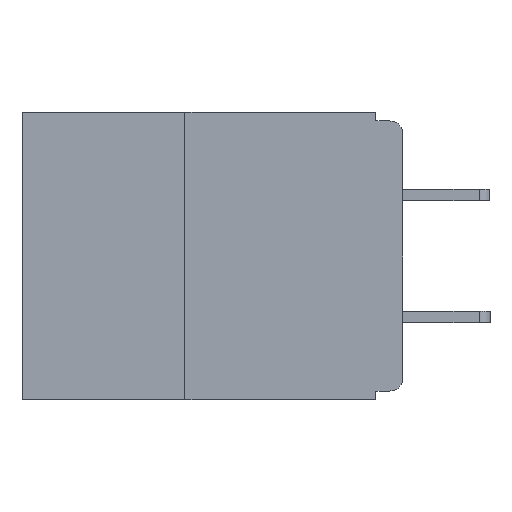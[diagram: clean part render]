
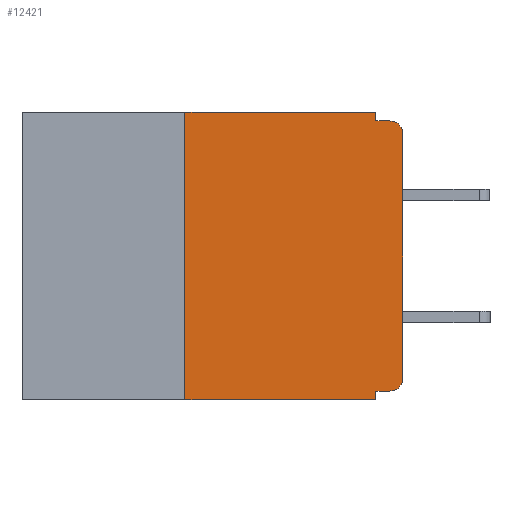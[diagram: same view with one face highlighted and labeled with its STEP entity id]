
A CAD part, left-side view. The second image highlights one B-rep face of the part: STEP entity #12421.
In plain terms, the highlighted planar face has unit normal (-1, 0, 0).
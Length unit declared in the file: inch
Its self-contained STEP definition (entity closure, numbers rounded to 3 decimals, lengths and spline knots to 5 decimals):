
#20 = ORIENTED_EDGE ( 'NONE', *, *, #16662, .T. ) ;
#504 = CARTESIAN_POINT ( 'NONE',  ( 0., 0., 0. ) ) ;
#861 = CARTESIAN_POINT ( 'NONE',  ( 0., 0., -0.025 ) ) ;
#1582 = ORIENTED_EDGE ( 'NONE', *, *, #31249, .T. ) ;
#1632 = VERTEX_POINT ( 'NONE', #21665 ) ;
#2095 = LINE ( 'NONE', #20295, #14384 ) ;
#2736 = AXIS2_PLACEMENT_3D ( 'NONE', #5740, #22915, #8243 ) ;
#3205 = CARTESIAN_POINT ( 'NONE',  ( 0., 0.031, -0.33 ) ) ;
#3583 = CARTESIAN_POINT ( 'NONE',  ( 0., 0.031, 0. ) ) ;
#3768 = VERTEX_POINT ( 'NONE', #4635 ) ;
#4081 = VECTOR ( 'NONE', #13681, 39.37008 ) ;
#4127 = DIRECTION ( 'NONE',  ( 0., 0., -1. ) ) ;
#4635 = CARTESIAN_POINT ( 'NONE',  ( 0., 0.015, -0.32 ) ) ;
#4846 = LINE ( 'NONE', #29127, #23642 ) ;
#5740 = CARTESIAN_POINT ( 'NONE',  ( 0., 0.015, -0.305 ) ) ;
#5940 = DIRECTION ( 'NONE',  ( 1., 0., 0. ) ) ;
#6138 = VERTEX_POINT ( 'NONE', #16312 ) ;
#6229 = CARTESIAN_POINT ( 'NONE',  ( 0., 0.015, -0.025 ) ) ;
#6965 = ORIENTED_EDGE ( 'NONE', *, *, #12370, .T. ) ;
#7021 = VERTEX_POINT ( 'NONE', #3205 ) ;
#7223 = FACE_OUTER_BOUND ( 'NONE', #7234, .T. ) ;
#7234 = EDGE_LOOP ( 'NONE', ( #1582, #16169, #7750, #20772, #28687, #18882, #20, #30564, #12710, #6965 ) ) ;
#7750 = ORIENTED_EDGE ( 'NONE', *, *, #13409, .F. ) ;
#8199 = EDGE_CURVE ( 'NONE', #6138, #17475, #31537, .T. ) ;
#8243 = DIRECTION ( 'NONE',  ( 0., 0., -1. ) ) ;
#8496 = LINE ( 'NONE', #3583, #25672 ) ;
#8737 = DIRECTION ( 'NONE',  ( 0., 0., -1. ) ) ;
#9565 = CIRCLE ( 'NONE', #2736, 0.015 ) ;
#9717 = VECTOR ( 'NONE', #4127, 39.37008 ) ;
#10098 = EDGE_CURVE ( 'NONE', #19013, #7021, #17009, .T. ) ;
#11985 = LINE ( 'NONE', #24478, #24993 ) ;
#12370 = EDGE_CURVE ( 'NONE', #3768, #24733, #9565, .T. ) ;
#12421 = ADVANCED_FACE ( 'NONE', ( #7223 ), #18208, .F. ) ;
#12710 = ORIENTED_EDGE ( 'NONE', *, *, #27077, .F. ) ;
#13221 = CARTESIAN_POINT ( 'NONE',  ( 0., 0.015, -0.01 ) ) ;
#13409 = EDGE_CURVE ( 'NONE', #1632, #30716, #4846, .T. ) ;
#13681 = DIRECTION ( 'NONE',  ( 0., -1., 0. ) ) ;
#14384 = VECTOR ( 'NONE', #22774, 39.37008 ) ;
#14956 = DIRECTION ( 'NONE',  ( 0., -1., 0. ) ) ;
#16169 = ORIENTED_EDGE ( 'NONE', *, *, #18958, .T. ) ;
#16205 = CARTESIAN_POINT ( 'NONE',  ( 0., 0.031, -0.32 ) ) ;
#16312 = CARTESIAN_POINT ( 'NONE',  ( 0., 0.25, 0. ) ) ;
#16662 = EDGE_CURVE ( 'NONE', #31439, #7021, #23657, .T. ) ;
#17009 = LINE ( 'NONE', #28443, #9717 ) ;
#17128 = DIRECTION ( 'NONE',  ( 0., 0., 1. ) ) ;
#17278 = VECTOR ( 'NONE', #17742, 39.37008 ) ;
#17475 = VERTEX_POINT ( 'NONE', #24228 ) ;
#17592 = AXIS2_PLACEMENT_3D ( 'NONE', #20644, #5940, #23116 ) ;
#17742 = DIRECTION ( 'NONE',  ( 0., 0., 1. ) ) ;
#18208 = PLANE ( 'NONE',  #17592 ) ;
#18221 = CARTESIAN_POINT ( 'NONE',  ( 0., 0., -0.305 ) ) ;
#18774 = VECTOR ( 'NONE', #14956, 39.37008 ) ;
#18882 = ORIENTED_EDGE ( 'NONE', *, *, #19933, .F. ) ;
#18958 = EDGE_CURVE ( 'NONE', #27129, #30716, #28365, .T. ) ;
#19013 = VERTEX_POINT ( 'NONE', #16205 ) ;
#19773 = CARTESIAN_POINT ( 'NONE',  ( 0., 0.437, 0. ) ) ;
#19933 = EDGE_CURVE ( 'NONE', #31439, #6138, #11985, .T. ) ;
#20295 = CARTESIAN_POINT ( 'NONE',  ( 0., 0., -0.32 ) ) ;
#20644 = CARTESIAN_POINT ( 'NONE',  ( 0., 0.437, 0. ) ) ;
#20747 = DIRECTION ( 'NONE',  ( 0., 0., -1. ) ) ;
#20772 = ORIENTED_EDGE ( 'NONE', *, *, #23218, .F. ) ;
#21665 = CARTESIAN_POINT ( 'NONE',  ( 0., 0.031, -0.01 ) ) ;
#22774 = DIRECTION ( 'NONE',  ( 0., 1., 0. ) ) ;
#22915 = DIRECTION ( 'NONE',  ( -1., 0., 0. ) ) ;
#23116 = DIRECTION ( 'NONE',  ( 0., 0., -1. ) ) ;
#23218 = EDGE_CURVE ( 'NONE', #17475, #1632, #8496, .T. ) ;
#23260 = CARTESIAN_POINT ( 'NONE',  ( 0., 0.25, -0.33 ) ) ;
#23377 = DIRECTION ( 'NONE',  ( -1., 0., 0. ) ) ;
#23642 = VECTOR ( 'NONE', #26746, 39.37008 ) ;
#23657 = LINE ( 'NONE', #25843, #4081 ) ;
#24228 = CARTESIAN_POINT ( 'NONE',  ( 0., 0.031, 0. ) ) ;
#24478 = CARTESIAN_POINT ( 'NONE',  ( 0., 0.25, -0.33 ) ) ;
#24510 = LINE ( 'NONE', #504, #17278 ) ;
#24733 = VERTEX_POINT ( 'NONE', #18221 ) ;
#24993 = VECTOR ( 'NONE', #17128, 39.37008 ) ;
#25672 = VECTOR ( 'NONE', #20747, 39.37008 ) ;
#25843 = CARTESIAN_POINT ( 'NONE',  ( 0., 0.437, -0.33 ) ) ;
#26041 = AXIS2_PLACEMENT_3D ( 'NONE', #6229, #23377, #8737 ) ;
#26746 = DIRECTION ( 'NONE',  ( 0., -1., 0. ) ) ;
#27077 = EDGE_CURVE ( 'NONE', #3768, #19013, #2095, .T. ) ;
#27129 = VERTEX_POINT ( 'NONE', #861 ) ;
#28365 = CIRCLE ( 'NONE', #26041, 0.015 ) ;
#28443 = CARTESIAN_POINT ( 'NONE',  ( 0., 0.031, -0.33 ) ) ;
#28687 = ORIENTED_EDGE ( 'NONE', *, *, #8199, .F. ) ;
#29127 = CARTESIAN_POINT ( 'NONE',  ( 0., 0., -0.01 ) ) ;
#30564 = ORIENTED_EDGE ( 'NONE', *, *, #10098, .F. ) ;
#30716 = VERTEX_POINT ( 'NONE', #13221 ) ;
#31249 = EDGE_CURVE ( 'NONE', #24733, #27129, #24510, .T. ) ;
#31439 = VERTEX_POINT ( 'NONE', #23260 ) ;
#31537 = LINE ( 'NONE', #19773, #18774 ) ;
